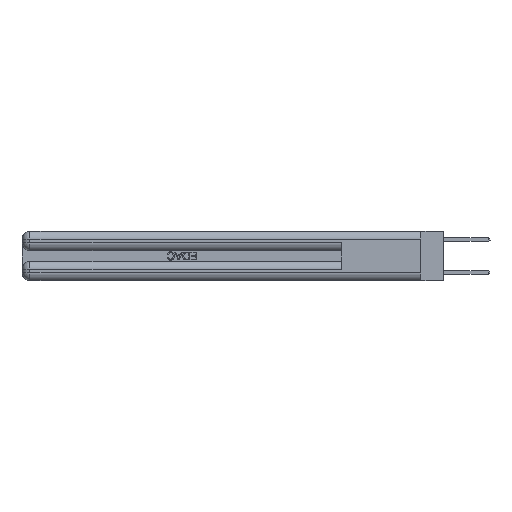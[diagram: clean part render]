
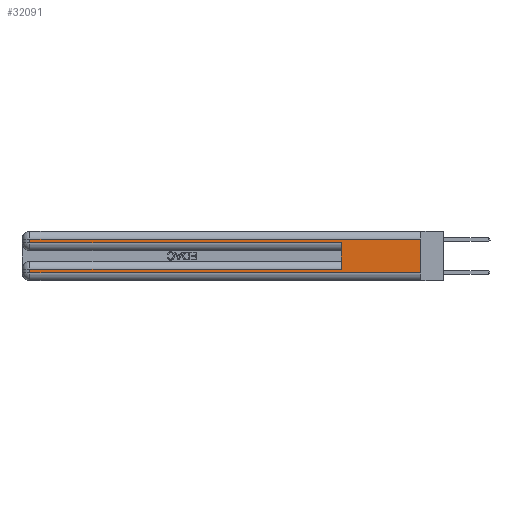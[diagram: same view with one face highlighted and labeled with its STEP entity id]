
A CAD part, left-side view. The second image highlights one B-rep face of the part: STEP entity #32091.
In plain terms, the highlighted planar face has unit normal (-1, 0, 0).
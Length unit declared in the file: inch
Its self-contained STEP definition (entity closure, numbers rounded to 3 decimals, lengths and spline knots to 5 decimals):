
#270 = LINE ( 'NONE', #8033, #24935 ) ;
#588 = EDGE_CURVE ( 'NONE', #16118, #1656, #24563, .T. ) ;
#627 = EDGE_CURVE ( 'NONE', #18489, #24321, #15243, .T. ) ;
#791 = ORIENTED_EDGE ( 'NONE', *, *, #9455, .T. ) ;
#1213 = ORIENTED_EDGE ( 'NONE', *, *, #588, .F. ) ;
#1656 = VERTEX_POINT ( 'NONE', #31014 ) ;
#1772 = DIRECTION ( 'NONE',  ( 0., -1., 0. ) ) ;
#1883 = CARTESIAN_POINT ( 'NONE',  ( 0., 0., 0.37 ) ) ;
#2332 = FACE_OUTER_BOUND ( 'NONE', #25025, .T. ) ;
#3258 = LINE ( 'NONE', #23627, #11767 ) ;
#5302 = DIRECTION ( 'NONE',  ( 0., 0., -1. ) ) ;
#5466 = VECTOR ( 'NONE', #29246, 39.37008 ) ;
#6558 = LINE ( 'NONE', #26767, #5466 ) ;
#7277 = ORIENTED_EDGE ( 'NONE', *, *, #16101, .T. ) ;
#8033 = CARTESIAN_POINT ( 'NONE',  ( 0., 0., 0.06 ) ) ;
#8896 = VERTEX_POINT ( 'NONE', #20808 ) ;
#9455 = EDGE_CURVE ( 'NONE', #16237, #1656, #270, .T. ) ;
#9498 = DIRECTION ( 'NONE',  ( 0., 0., -1. ) ) ;
#10499 = VERTEX_POINT ( 'NONE', #24803 ) ;
#11047 = CARTESIAN_POINT ( 'NONE',  ( 0., 0., 0.31 ) ) ;
#11767 = VECTOR ( 'NONE', #16355, 39.37008 ) ;
#11907 = VECTOR ( 'NONE', #5302, 39.37008 ) ;
#11941 = CARTESIAN_POINT ( 'NONE',  ( 0., 0., 0.31 ) ) ;
#12026 = CARTESIAN_POINT ( 'NONE',  ( 0., 0., 0.285 ) ) ;
#13030 = VECTOR ( 'NONE', #27506, 39.37008 ) ;
#14370 = LINE ( 'NONE', #12026, #31914 ) ;
#14534 = CARTESIAN_POINT ( 'NONE',  ( 0., 2.94, 0.06 ) ) ;
#14961 = VERTEX_POINT ( 'NONE', #26882 ) ;
#15191 = CARTESIAN_POINT ( 'NONE',  ( 0., 0.6, 0.285 ) ) ;
#15243 = LINE ( 'NONE', #30927, #25727 ) ;
#16061 = CARTESIAN_POINT ( 'NONE',  ( 0., 0., 0.37 ) ) ;
#16101 = EDGE_CURVE ( 'NONE', #14961, #16237, #3258, .T. ) ;
#16118 = VERTEX_POINT ( 'NONE', #11047 ) ;
#16237 = VERTEX_POINT ( 'NONE', #14534 ) ;
#16355 = DIRECTION ( 'NONE',  ( 0., 0., -1. ) ) ;
#18054 = CARTESIAN_POINT ( 'NONE',  ( 0., 2.94, 0.37 ) ) ;
#18140 = DIRECTION ( 'NONE',  ( 0., -1., 0. ) ) ;
#18489 = VERTEX_POINT ( 'NONE', #24557 ) ;
#18869 = PLANE ( 'NONE',  #28825 ) ;
#19739 = ORIENTED_EDGE ( 'NONE', *, *, #30332, .T. ) ;
#20678 = LINE ( 'NONE', #18054, #11907 ) ;
#20808 = CARTESIAN_POINT ( 'NONE',  ( 0., 2.94, 0.285 ) ) ;
#20971 = VECTOR ( 'NONE', #9498, 39.37008 ) ;
#21311 = ORIENTED_EDGE ( 'NONE', *, *, #22205, .T. ) ;
#21511 = DIRECTION ( 'NONE',  ( 0., 0., -1. ) ) ;
#22018 = ORIENTED_EDGE ( 'NONE', *, *, #627, .F. ) ;
#22205 = EDGE_CURVE ( 'NONE', #16118, #10499, #30305, .T. ) ;
#22991 = DIRECTION ( 'NONE',  ( 0., 0., 1. ) ) ;
#23627 = CARTESIAN_POINT ( 'NONE',  ( 0., 2.94, 0.37 ) ) ;
#24321 = VERTEX_POINT ( 'NONE', #15191 ) ;
#24557 = CARTESIAN_POINT ( 'NONE',  ( 0., 0.6, 0.085 ) ) ;
#24563 = LINE ( 'NONE', #1883, #20971 ) ;
#24803 = CARTESIAN_POINT ( 'NONE',  ( 0., 2.94, 0.31 ) ) ;
#24935 = VECTOR ( 'NONE', #18140, 39.37008 ) ;
#25025 = EDGE_LOOP ( 'NONE', ( #1213, #21311, #27083, #19739, #22018, #28560, #7277, #791 ) ) ;
#25727 = VECTOR ( 'NONE', #22991, 39.37008 ) ;
#26767 = CARTESIAN_POINT ( 'NONE',  ( 0., 0., 0.085 ) ) ;
#26882 = CARTESIAN_POINT ( 'NONE',  ( 0., 2.94, 0.085 ) ) ;
#27083 = ORIENTED_EDGE ( 'NONE', *, *, #32066, .T. ) ;
#27506 = DIRECTION ( 'NONE',  ( 0., 1., 0. ) ) ;
#28560 = ORIENTED_EDGE ( 'NONE', *, *, #30208, .T. ) ;
#28825 = AXIS2_PLACEMENT_3D ( 'NONE', #16061, #30945, #21511 ) ;
#29246 = DIRECTION ( 'NONE',  ( 0., 1., 0. ) ) ;
#30208 = EDGE_CURVE ( 'NONE', #18489, #14961, #6558, .T. ) ;
#30305 = LINE ( 'NONE', #11941, #13030 ) ;
#30332 = EDGE_CURVE ( 'NONE', #8896, #24321, #14370, .T. ) ;
#30927 = CARTESIAN_POINT ( 'NONE',  ( 0., 0.6, 0.145 ) ) ;
#30945 = DIRECTION ( 'NONE',  ( 1., 0., 0. ) ) ;
#31014 = CARTESIAN_POINT ( 'NONE',  ( 0., 0., 0.06 ) ) ;
#31914 = VECTOR ( 'NONE', #1772, 39.37008 ) ;
#32066 = EDGE_CURVE ( 'NONE', #10499, #8896, #20678, .T. ) ;
#32091 = ADVANCED_FACE ( 'NONE', ( #2332 ), #18869, .F. ) ;
